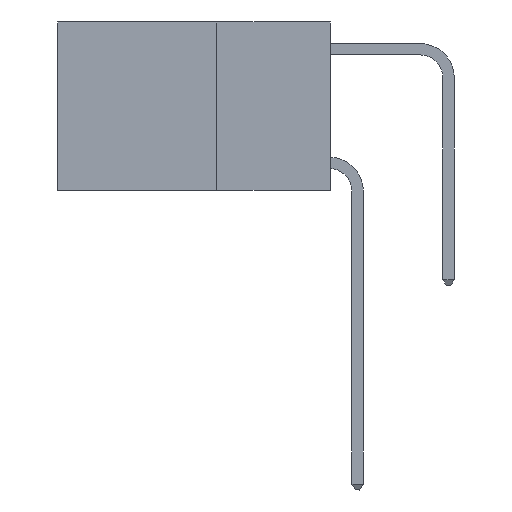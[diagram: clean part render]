
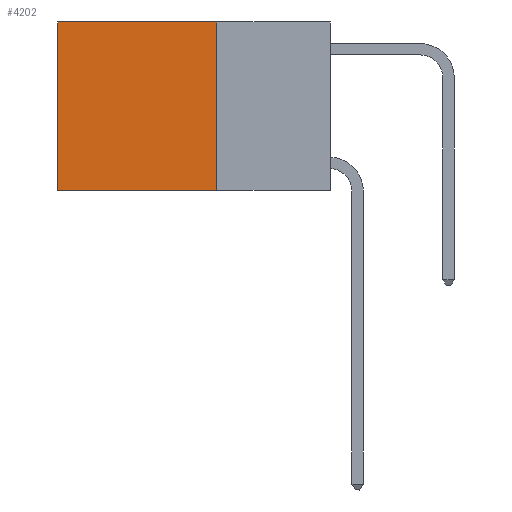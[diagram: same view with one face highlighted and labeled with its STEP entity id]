
A CAD part, left-side view. The second image highlights one B-rep face of the part: STEP entity #4202.
In plain terms, the highlighted planar face has unit normal (-1, 0, 0).
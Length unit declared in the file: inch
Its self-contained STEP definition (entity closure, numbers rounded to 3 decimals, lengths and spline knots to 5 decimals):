
#10 = DIRECTION ( 'NONE',  ( 0., 0., -1. ) ) ;
#232 = VERTEX_POINT ( 'NONE', #11159 ) ;
#327 = CARTESIAN_POINT ( 'NONE',  ( 0.2625, 0.25, -0.37 ) ) ;
#746 = CARTESIAN_POINT ( 'NONE',  ( 0.2625, 0.6, -0.37 ) ) ;
#1089 = EDGE_CURVE ( 'NONE', #3216, #3874, #4097, .T. ) ;
#1272 = DIRECTION ( 'NONE',  ( 0., 1., 0. ) ) ;
#1292 = ORIENTED_EDGE ( 'NONE', *, *, #1089, .T. ) ;
#1561 = LINE ( 'NONE', #327, #12051 ) ;
#2201 = ORIENTED_EDGE ( 'NONE', *, *, #10582, .T. ) ;
#3188 = ORIENTED_EDGE ( 'NONE', *, *, #7392, .F. ) ;
#3216 = VERTEX_POINT ( 'NONE', #5342 ) ;
#3429 = VECTOR ( 'NONE', #1272, 39.37008 ) ;
#3831 = PLANE ( 'NONE',  #8402 ) ;
#3874 = VERTEX_POINT ( 'NONE', #13209 ) ;
#4097 = LINE ( 'NONE', #10546, #3429 ) ;
#4202 = ADVANCED_FACE ( 'NONE', ( #6548 ), #3831, .F. ) ;
#4807 = ORIENTED_EDGE ( 'NONE', *, *, #8581, .F. ) ;
#4982 = VECTOR ( 'NONE', #7707, 39.37008 ) ;
#5342 = CARTESIAN_POINT ( 'NONE',  ( 0.2625, 0.25, 0. ) ) ;
#5818 = DIRECTION ( 'NONE',  ( 0., 0., -1. ) ) ;
#6548 = FACE_OUTER_BOUND ( 'NONE', #6668, .T. ) ;
#6668 = EDGE_LOOP ( 'NONE', ( #2201, #4807, #3188, #1292 ) ) ;
#7392 = EDGE_CURVE ( 'NONE', #3216, #232, #10848, .T. ) ;
#7707 = DIRECTION ( 'NONE',  ( 0., 0., -1. ) ) ;
#8402 = AXIS2_PLACEMENT_3D ( 'NONE', #8734, #12568, #5818 ) ;
#8581 = EDGE_CURVE ( 'NONE', #232, #8831, #1561, .T. ) ;
#8734 = CARTESIAN_POINT ( 'NONE',  ( 0.2625, 0.25, 0. ) ) ;
#8831 = VERTEX_POINT ( 'NONE', #746 ) ;
#10186 = LINE ( 'NONE', #12484, #4982 ) ;
#10546 = CARTESIAN_POINT ( 'NONE',  ( 0.2625, 0.25, 0. ) ) ;
#10582 = EDGE_CURVE ( 'NONE', #3874, #8831, #10186, .T. ) ;
#10592 = CARTESIAN_POINT ( 'NONE',  ( 0.2625, 0.25, 0. ) ) ;
#10848 = LINE ( 'NONE', #10592, #12820 ) ;
#11159 = CARTESIAN_POINT ( 'NONE',  ( 0.2625, 0.25, -0.37 ) ) ;
#12051 = VECTOR ( 'NONE', #12731, 39.37008 ) ;
#12484 = CARTESIAN_POINT ( 'NONE',  ( 0.2625, 0.6, 0. ) ) ;
#12568 = DIRECTION ( 'NONE',  ( 1., 0., 0. ) ) ;
#12731 = DIRECTION ( 'NONE',  ( 0., 1., 0. ) ) ;
#12820 = VECTOR ( 'NONE', #10, 39.37008 ) ;
#13209 = CARTESIAN_POINT ( 'NONE',  ( 0.2625, 0.6, 0. ) ) ;
